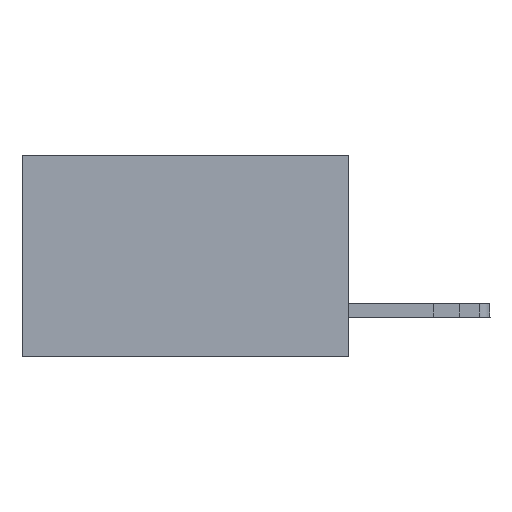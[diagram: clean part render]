
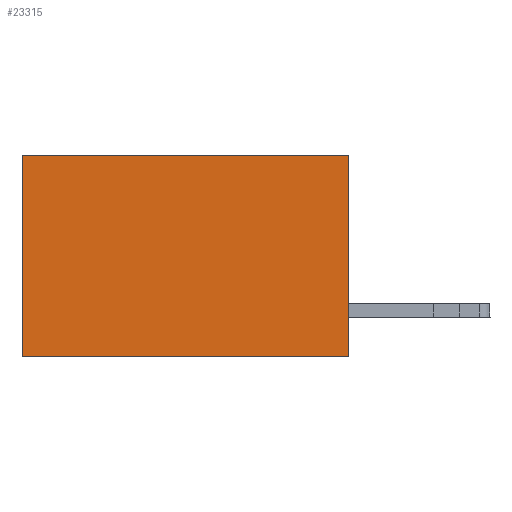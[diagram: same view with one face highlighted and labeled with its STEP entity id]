
A CAD part, left-side view. The second image highlights one B-rep face of the part: STEP entity #23315.
In plain terms, the highlighted planar face has unit normal (-1, 0, 0).
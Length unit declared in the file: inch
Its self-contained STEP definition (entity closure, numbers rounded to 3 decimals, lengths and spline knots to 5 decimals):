
#383 = VERTEX_POINT ( 'NONE', #5726 ) ;
#1295 = CARTESIAN_POINT ( 'NONE',  ( 0.298, 0.6, 0. ) ) ;
#3441 = LINE ( 'NONE', #22847, #18166 ) ;
#4056 = DIRECTION ( 'NONE',  ( 0., 0., -1. ) ) ;
#4103 = ORIENTED_EDGE ( 'NONE', *, *, #17762, .T. ) ;
#4456 = AXIS2_PLACEMENT_3D ( 'NONE', #19196, #21199, #4056 ) ;
#5251 = EDGE_LOOP ( 'NONE', ( #12580, #8368, #10364, #4103 ) ) ;
#5726 = CARTESIAN_POINT ( 'NONE',  ( 0.298, 0., -0.37 ) ) ;
#5771 = CARTESIAN_POINT ( 'NONE',  ( 0.298, 0., -0.37 ) ) ;
#8368 = ORIENTED_EDGE ( 'NONE', *, *, #8694, .F. ) ;
#8694 = EDGE_CURVE ( 'NONE', #383, #21341, #20799, .T. ) ;
#10364 = ORIENTED_EDGE ( 'NONE', *, *, #12862, .F. ) ;
#11131 = VECTOR ( 'NONE', #14424, 39.37008 ) ;
#11197 = DIRECTION ( 'NONE',  ( 0., 0., -1. ) ) ;
#11561 = PLANE ( 'NONE',  #4456 ) ;
#12580 = ORIENTED_EDGE ( 'NONE', *, *, #19967, .T. ) ;
#12862 = EDGE_CURVE ( 'NONE', #17319, #383, #3441, .T. ) ;
#13069 = FACE_OUTER_BOUND ( 'NONE', #5251, .T. ) ;
#13112 = LINE ( 'NONE', #24119, #19611 ) ;
#14058 = LINE ( 'NONE', #23800, #11131 ) ;
#14424 = DIRECTION ( 'NONE',  ( 0., 1., 0. ) ) ;
#15569 = VERTEX_POINT ( 'NONE', #1295 ) ;
#17319 = VERTEX_POINT ( 'NONE', #24208 ) ;
#17762 = EDGE_CURVE ( 'NONE', #17319, #15569, #14058, .T. ) ;
#18166 = VECTOR ( 'NONE', #11197, 39.37008 ) ;
#18363 = DIRECTION ( 'NONE',  ( 0., 0., -1. ) ) ;
#19196 = CARTESIAN_POINT ( 'NONE',  ( 0.298, 0., 0. ) ) ;
#19611 = VECTOR ( 'NONE', #18363, 39.37008 ) ;
#19967 = EDGE_CURVE ( 'NONE', #15569, #21341, #13112, .T. ) ;
#20799 = LINE ( 'NONE', #5771, #24083 ) ;
#21199 = DIRECTION ( 'NONE',  ( 1., 0., 0. ) ) ;
#21341 = VERTEX_POINT ( 'NONE', #24222 ) ;
#22847 = CARTESIAN_POINT ( 'NONE',  ( 0.298, 0., 0. ) ) ;
#23043 = DIRECTION ( 'NONE',  ( 0., 1., 0. ) ) ;
#23315 = ADVANCED_FACE ( 'NONE', ( #13069 ), #11561, .F. ) ;
#23800 = CARTESIAN_POINT ( 'NONE',  ( 0.298, 0., 0. ) ) ;
#24083 = VECTOR ( 'NONE', #23043, 39.37008 ) ;
#24119 = CARTESIAN_POINT ( 'NONE',  ( 0.298, 0.6, 0. ) ) ;
#24208 = CARTESIAN_POINT ( 'NONE',  ( 0.298, 0., 0. ) ) ;
#24222 = CARTESIAN_POINT ( 'NONE',  ( 0.298, 0.6, -0.37 ) ) ;
